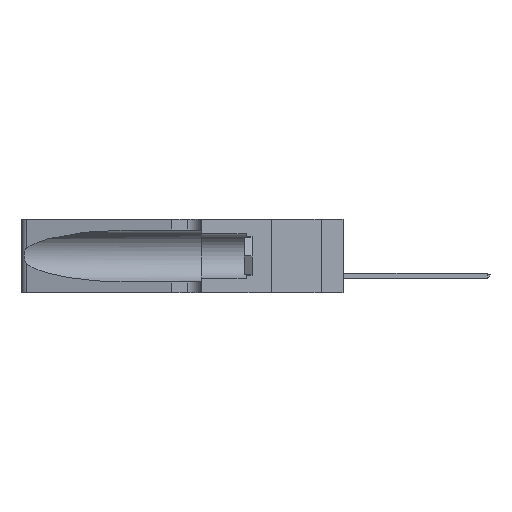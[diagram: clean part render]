
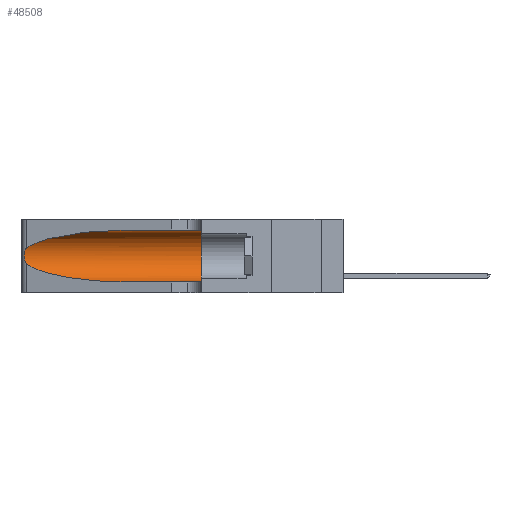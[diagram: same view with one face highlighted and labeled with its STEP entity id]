
A CAD part, left-side view. The second image highlights one B-rep face of the part: STEP entity #48508.
In plain terms, the highlighted cylindrical face has radius 3.308 mm (diameter 6.617 mm), a partial arc.
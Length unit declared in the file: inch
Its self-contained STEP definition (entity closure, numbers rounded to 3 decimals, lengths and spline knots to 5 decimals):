
#476 = CARTESIAN_POINT ( 'NONE',  ( 0.1305, 0.35, 0.185 ) ) ;
#827 = CYLINDRICAL_SURFACE ( 'NONE', #14091, 0.13025 ) ;
#1324 = CARTESIAN_POINT ( 'NONE',  ( 0.1305, 0.72297, 0.05475 ) ) ;
#1461 = DIRECTION ( 'NONE',  ( 0., 1., 0. ) ) ;
#2121 = DIRECTION ( 'NONE',  ( 0., -1., 0. ) ) ;
#3261 = ORIENTED_EDGE ( 'NONE', *, *, #20218, .T. ) ;
#4080 = CARTESIAN_POINT ( 'NONE',  ( 0.25639, 1.23186, 0.15144 ) ) ;
#4602 = CARTESIAN_POINT ( 'NONE',  ( 0.26075, 1.23896, 0.19203 ) ) ;
#9121 = CARTESIAN_POINT ( 'NONE',  ( 0.26017, 1.23833, 0.17102 ) ) ;
#9999 = LINE ( 'NONE', #11228, #26073 ) ;
#10278 = ORIENTED_EDGE ( 'NONE', *, *, #32287, .T. ) ;
#11094 = CIRCLE ( 'NONE', #18170, 0.13025 ) ;
#11228 = CARTESIAN_POINT ( 'NONE',  ( 0.1305, 1.61858, 0.05475 ) ) ;
#11935 = CARTESIAN_POINT ( 'NONE',  ( 0.25555, 1.22994, 0.2215 ) ) ;
#12074 = VERTEX_POINT ( 'NONE', #25738 ) ;
#12393 = CARTESIAN_POINT ( 'NONE',  ( 0.25854, 1.2359, 0.20912 ) ) ;
#13159 = EDGE_CURVE ( 'NONE', #21826, #22519, #44401, .T. ) ;
#14091 = AXIS2_PLACEMENT_3D ( 'NONE', #40384, #2121, #35880 ) ;
#15901 = CARTESIAN_POINT ( 'NONE',  ( 0.25639, 1.23184, 0.21858 ) ) ;
#15991 = ORIENTED_EDGE ( 'NONE', *, *, #27528, .T. ) ;
#16138 = CARTESIAN_POINT ( 'NONE',  ( 0.26075, 1.23896, 0.178 ) ) ;
#17025 = VERTEX_POINT ( 'NONE', #1324 ) ;
#18170 = AXIS2_PLACEMENT_3D ( 'NONE', #476, #1461, #35229 ) ;
#18189 = CARTESIAN_POINT ( 'NONE',  ( 0.25789, 1.23486, 0.15765 ) ) ;
#18959 = VERTEX_POINT ( 'NONE', #40531 ) ;
#19501 = CARTESIAN_POINT ( 'NONE',  ( 0.1305, 0.72297, 0.31525 ) ) ;
#20218 = EDGE_CURVE ( 'NONE', #12074, #17025, #35465, .T. ) ;
#21007 = CARTESIAN_POINT ( 'NONE',  ( 0.1305, 0.35, 0.05475 ) ) ;
#21184 = CARTESIAN_POINT ( 'NONE',  ( 0.25487, 1.22718, 0.14631 ) ) ;
#21826 = VERTEX_POINT ( 'NONE', #28102 ) ;
#22519 = VERTEX_POINT ( 'NONE', #28094 ) ;
#23034 = VERTEX_POINT ( 'NONE', #21007 ) ;
#23094 = CARTESIAN_POINT ( 'NONE',  ( 0.25487, 1.22718, 0.14631 ) ) ;
#23220 = CARTESIAN_POINT ( 'NONE',  ( 0.1305, 1.61858, 0.31525 ) ) ;
#25170 = CARTESIAN_POINT ( 'NONE',  ( 0.18966, 0.96281, 0.05475 ) ) ;
#25455 = CARTESIAN_POINT ( 'NONE',  ( 0.25856, 1.23593, 0.16098 ) ) ;
#25738 = CARTESIAN_POINT ( 'NONE',  ( 0.25487, 1.22718, 0.14631 ) ) ;
#26073 = VECTOR ( 'NONE', #49181, 39.37008 ) ;
#27528 = EDGE_CURVE ( 'NONE', #21826, #18959, #43161, .T. ) ;
#27695 = CARTESIAN_POINT ( 'NONE',  ( 0.2373, 1.15595, 0.08982 ) ) ;
#28094 = CARTESIAN_POINT ( 'NONE',  ( 0.1305, 0.35, 0.31525 ) ) ;
#28102 = CARTESIAN_POINT ( 'NONE',  ( 0.1305, 0.72297, 0.31525 ) ) ;
#28469 = ORIENTED_EDGE ( 'NONE', *, *, #13159, .F. ) ;
#30278 = EDGE_CURVE ( 'NONE', #18959, #12074, #43818, .T. ) ;
#31015 = CARTESIAN_POINT ( 'NONE',  ( 0.25487, 1.22718, 0.22369 ) ) ;
#31306 = VECTOR ( 'NONE', #43413, 39.37008 ) ;
#32287 = EDGE_CURVE ( 'NONE', #17025, #23034, #9999, .T. ) ;
#33229 = ORIENTED_EDGE ( 'NONE', *, *, #33840, .F. ) ;
#33369 = CARTESIAN_POINT ( 'NONE',  ( 0.1305, 0.72297, 0.05475 ) ) ;
#33840 = EDGE_CURVE ( 'NONE', #22519, #23034, #11094, .T. ) ;
#34195 = CARTESIAN_POINT ( 'NONE',  ( 0.25555, 1.22993, 0.14849 ) ) ;
#35043 = CARTESIAN_POINT ( 'NONE',  ( 0.18966, 0.96281, 0.31525 ) ) ;
#35229 = DIRECTION ( 'NONE',  ( 0., 0., 1. ) ) ;
#35465 =( BOUNDED_CURVE ( )  B_SPLINE_CURVE ( 3, ( #21184, #27695, #25170, #33369 ),
 .UNSPECIFIED., .F., .F. ) 
 B_SPLINE_CURVE_WITH_KNOTS ( ( 4, 4 ),
 ( 3.44316, 4.71239 ),
 .UNSPECIFIED. ) 
 CURVE ( )  GEOMETRIC_REPRESENTATION_ITEM ( )  RATIONAL_B_SPLINE_CURVE ( ( 1., 0.87, 0.87, 1. ) ) 
 REPRESENTATION_ITEM ( '' )  );
#35880 = DIRECTION ( 'NONE',  ( 0., 0., -1. ) ) ;
#36879 = CARTESIAN_POINT ( 'NONE',  ( 0.26018, 1.23835, 0.19895 ) ) ;
#38711 = CARTESIAN_POINT ( 'NONE',  ( 0.2373, 1.15595, 0.28018 ) ) ;
#40384 = CARTESIAN_POINT ( 'NONE',  ( 0.1305, 1.61858, 0.185 ) ) ;
#40531 = CARTESIAN_POINT ( 'NONE',  ( 0.25487, 1.22718, 0.22369 ) ) ;
#42498 = CARTESIAN_POINT ( 'NONE',  ( 0.25487, 1.22718, 0.22369 ) ) ;
#42840 = EDGE_LOOP ( 'NONE', ( #15991, #46960, #3261, #10278, #33229, #28469 ) ) ;
#43161 =( BOUNDED_CURVE ( )  B_SPLINE_CURVE ( 3, ( #19501, #35043, #38711, #42498 ),
 .UNSPECIFIED., .F., .F. ) 
 B_SPLINE_CURVE_WITH_KNOTS ( ( 4, 4 ),
 ( 1.5708, 2.84003 ),
 .UNSPECIFIED. ) 
 CURVE ( )  GEOMETRIC_REPRESENTATION_ITEM ( )  RATIONAL_B_SPLINE_CURVE ( ( 1., 0.87, 0.87, 1. ) ) 
 REPRESENTATION_ITEM ( '' )  );
#43413 = DIRECTION ( 'NONE',  ( 0., -1., 0. ) ) ;
#43818 = B_SPLINE_CURVE_WITH_KNOTS ( 'NONE', 3,
 ( #31015, #11935, #15901, #46231, #12393, #36879, #4602, #16138, #9121, #25455, #18189, #4080, #34195, #23094 ),
 .UNSPECIFIED., .F., .F.,
 ( 4, 2, 2, 2, 2, 2, 4 ),
 ( 0., 0.00027, 0.00053, 0.00107, 0.0016, 0.00187, 0.00214 ),
 .UNSPECIFIED. ) ;
#44401 = LINE ( 'NONE', #23220, #31306 ) ;
#46026 = FACE_OUTER_BOUND ( 'NONE', #42840, .T. ) ;
#46231 = CARTESIAN_POINT ( 'NONE',  ( 0.25787, 1.23484, 0.2124 ) ) ;
#46960 = ORIENTED_EDGE ( 'NONE', *, *, #30278, .T. ) ;
#48508 = ADVANCED_FACE ( 'NONE', ( #46026 ), #827, .F. ) ;
#49181 = DIRECTION ( 'NONE',  ( 0., -1., 0. ) ) ;
